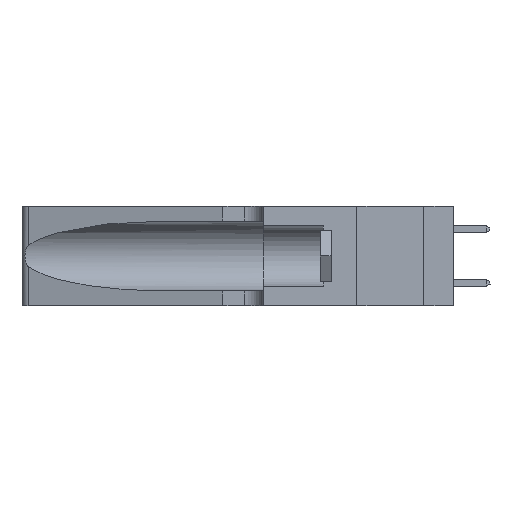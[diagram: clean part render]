
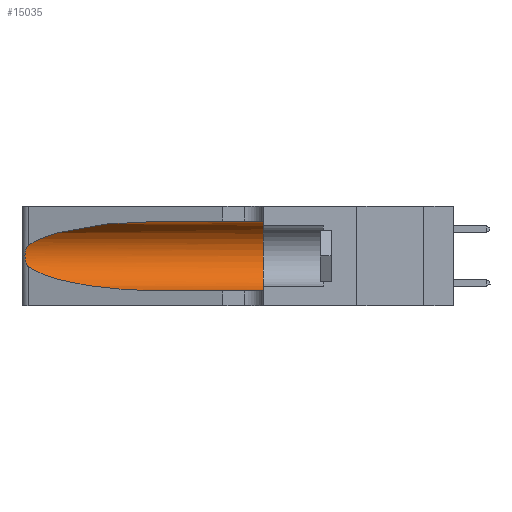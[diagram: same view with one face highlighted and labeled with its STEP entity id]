
A CAD part, left-side view. The second image highlights one B-rep face of the part: STEP entity #15035.
In plain terms, the highlighted cylindrical face has radius 3.308 mm (diameter 6.617 mm), a partial arc.
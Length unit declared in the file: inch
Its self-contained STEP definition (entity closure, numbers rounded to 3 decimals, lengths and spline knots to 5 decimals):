
#163 = VERTEX_POINT ( 'NONE', #3480 ) ;
#173 = AXIS2_PLACEMENT_3D ( 'NONE', #9687, #780, #11157 ) ;
#525 = CARTESIAN_POINT ( 'NONE',  ( 0.26017, 1.23833, 0.17102 ) ) ;
#617 = CARTESIAN_POINT ( 'NONE',  ( 0.1305, 0.72297, 0.31525 ) ) ;
#780 = DIRECTION ( 'NONE',  ( 0., 1., 0. ) ) ;
#1365 = CARTESIAN_POINT ( 'NONE',  ( 0.1305, 0.72297, 0.05475 ) ) ;
#1949 = CARTESIAN_POINT ( 'NONE',  ( 0.1305, 1.61858, 0.05475 ) ) ;
#2069 = CARTESIAN_POINT ( 'NONE',  ( 0.25789, 1.23486, 0.15765 ) ) ;
#2080 = LINE ( 'NONE', #1949, #9500 ) ;
#2328 = CYLINDRICAL_SURFACE ( 'NONE', #12852, 0.13025 ) ;
#2696 = VERTEX_POINT ( 'NONE', #1365 ) ;
#2714 = DIRECTION ( 'NONE',  ( 0., 0., -1. ) ) ;
#2957 = VERTEX_POINT ( 'NONE', #6389 ) ;
#3262 = VERTEX_POINT ( 'NONE', #10051 ) ;
#3333 = B_SPLINE_CURVE_WITH_KNOTS ( 'NONE', 3,
 ( #3544, #5078, #15253, #6555, #16700, #8006, #18146, #9458, #525, #10941, #2069, #12377, #3607, #13862 ),
 .UNSPECIFIED., .F., .F.,
 ( 4, 2, 2, 2, 2, 2, 4 ),
 ( 0., 0.00027, 0.00053, 0.00107, 0.0016, 0.00187, 0.00214 ),
 .UNSPECIFIED. ) ;
#3480 = CARTESIAN_POINT ( 'NONE',  ( 0.25487, 1.22718, 0.14631 ) ) ;
#3544 = CARTESIAN_POINT ( 'NONE',  ( 0.25487, 1.22718, 0.22369 ) ) ;
#3607 = CARTESIAN_POINT ( 'NONE',  ( 0.25555, 1.22993, 0.14849 ) ) ;
#5078 = CARTESIAN_POINT ( 'NONE',  ( 0.25555, 1.22994, 0.2215 ) ) ;
#5227 = CARTESIAN_POINT ( 'NONE',  ( 0.18966, 0.96281, 0.31525 ) ) ;
#6389 = CARTESIAN_POINT ( 'NONE',  ( 0.25487, 1.22718, 0.22369 ) ) ;
#6400 = ORIENTED_EDGE ( 'NONE', *, *, #11929, .T. ) ;
#6432 = ORIENTED_EDGE ( 'NONE', *, *, #15031, .F. ) ;
#6435 = EDGE_LOOP ( 'NONE', ( #10283, #9557, #6400, #15039, #18628, #6432 ) ) ;
#6555 = CARTESIAN_POINT ( 'NONE',  ( 0.25787, 1.23484, 0.2124 ) ) ;
#6701 = CARTESIAN_POINT ( 'NONE',  ( 0.25487, 1.22718, 0.22369 ) ) ;
#7477 = CARTESIAN_POINT ( 'NONE',  ( 0.18966, 0.96281, 0.05475 ) ) ;
#8006 = CARTESIAN_POINT ( 'NONE',  ( 0.26018, 1.23835, 0.19895 ) ) ;
#8217 =( BOUNDED_CURVE ( )  B_SPLINE_CURVE ( 3, ( #617, #5227, #15401, #6701 ),
 .UNSPECIFIED., .F., .F. ) 
 B_SPLINE_CURVE_WITH_KNOTS ( ( 4, 4 ),
 ( 1.5708, 2.84003 ),
 .UNSPECIFIED. ) 
 CURVE ( )  GEOMETRIC_REPRESENTATION_ITEM ( )  RATIONAL_B_SPLINE_CURVE ( ( 1., 0.87, 0.87, 1. ) ) 
 REPRESENTATION_ITEM ( '' )  );
#9458 = CARTESIAN_POINT ( 'NONE',  ( 0.26075, 1.23896, 0.178 ) ) ;
#9474 = CARTESIAN_POINT ( 'NONE',  ( 0.1305, 0.35, 0.31525 ) ) ;
#9500 = VECTOR ( 'NONE', #12267, 39.37008 ) ;
#9557 = ORIENTED_EDGE ( 'NONE', *, *, #10164, .T. ) ;
#9687 = CARTESIAN_POINT ( 'NONE',  ( 0.1305, 0.35, 0.185 ) ) ;
#9885 = VERTEX_POINT ( 'NONE', #14435 ) ;
#10051 = CARTESIAN_POINT ( 'NONE',  ( 0.1305, 0.72297, 0.31525 ) ) ;
#10094 = CARTESIAN_POINT ( 'NONE',  ( 0.1305, 1.61858, 0.31525 ) ) ;
#10164 = EDGE_CURVE ( 'NONE', #2957, #163, #3333, .T. ) ;
#10206 = FACE_OUTER_BOUND ( 'NONE', #6435, .T. ) ;
#10283 = ORIENTED_EDGE ( 'NONE', *, *, #16087, .T. ) ;
#10941 = CARTESIAN_POINT ( 'NONE',  ( 0.25856, 1.23593, 0.16098 ) ) ;
#11157 = DIRECTION ( 'NONE',  ( 0., 0., 1. ) ) ;
#11556 = CARTESIAN_POINT ( 'NONE',  ( 0.1305, 1.61858, 0.185 ) ) ;
#11929 = EDGE_CURVE ( 'NONE', #163, #2696, #13575, .T. ) ;
#12267 = DIRECTION ( 'NONE',  ( 0., -1., 0. ) ) ;
#12377 = CARTESIAN_POINT ( 'NONE',  ( 0.25639, 1.23186, 0.15144 ) ) ;
#12816 = VERTEX_POINT ( 'NONE', #9474 ) ;
#12852 = AXIS2_PLACEMENT_3D ( 'NONE', #11556, #15862, #2714 ) ;
#13276 = CARTESIAN_POINT ( 'NONE',  ( 0.25487, 1.22718, 0.14631 ) ) ;
#13575 =( BOUNDED_CURVE ( )  B_SPLINE_CURVE ( 3, ( #13276, #14727, #7477, #17638 ),
 .UNSPECIFIED., .F., .F. ) 
 B_SPLINE_CURVE_WITH_KNOTS ( ( 4, 4 ),
 ( 3.44316, 4.71239 ),
 .UNSPECIFIED. ) 
 CURVE ( )  GEOMETRIC_REPRESENTATION_ITEM ( )  RATIONAL_B_SPLINE_CURVE ( ( 1., 0.87, 0.87, 1. ) ) 
 REPRESENTATION_ITEM ( '' )  );
#13592 = CIRCLE ( 'NONE', #173, 0.13025 ) ;
#13862 = CARTESIAN_POINT ( 'NONE',  ( 0.25487, 1.22718, 0.14631 ) ) ;
#14435 = CARTESIAN_POINT ( 'NONE',  ( 0.1305, 0.35, 0.05475 ) ) ;
#14534 = LINE ( 'NONE', #10094, #17908 ) ;
#14727 = CARTESIAN_POINT ( 'NONE',  ( 0.2373, 1.15595, 0.08982 ) ) ;
#15031 = EDGE_CURVE ( 'NONE', #3262, #12816, #14534, .T. ) ;
#15035 = ADVANCED_FACE ( 'NONE', ( #10206 ), #2328, .F. ) ;
#15039 = ORIENTED_EDGE ( 'NONE', *, *, #15989, .T. ) ;
#15253 = CARTESIAN_POINT ( 'NONE',  ( 0.25639, 1.23184, 0.21858 ) ) ;
#15401 = CARTESIAN_POINT ( 'NONE',  ( 0.2373, 1.15595, 0.28018 ) ) ;
#15509 = EDGE_CURVE ( 'NONE', #12816, #9885, #13592, .T. ) ;
#15862 = DIRECTION ( 'NONE',  ( 0., -1., 0. ) ) ;
#15989 = EDGE_CURVE ( 'NONE', #2696, #9885, #2080, .T. ) ;
#16087 = EDGE_CURVE ( 'NONE', #3262, #2957, #8217, .T. ) ;
#16700 = CARTESIAN_POINT ( 'NONE',  ( 0.25854, 1.2359, 0.20912 ) ) ;
#17317 = DIRECTION ( 'NONE',  ( 0., -1., 0. ) ) ;
#17638 = CARTESIAN_POINT ( 'NONE',  ( 0.1305, 0.72297, 0.05475 ) ) ;
#17908 = VECTOR ( 'NONE', #17317, 39.37008 ) ;
#18146 = CARTESIAN_POINT ( 'NONE',  ( 0.26075, 1.23896, 0.19203 ) ) ;
#18628 = ORIENTED_EDGE ( 'NONE', *, *, #15509, .F. ) ;
